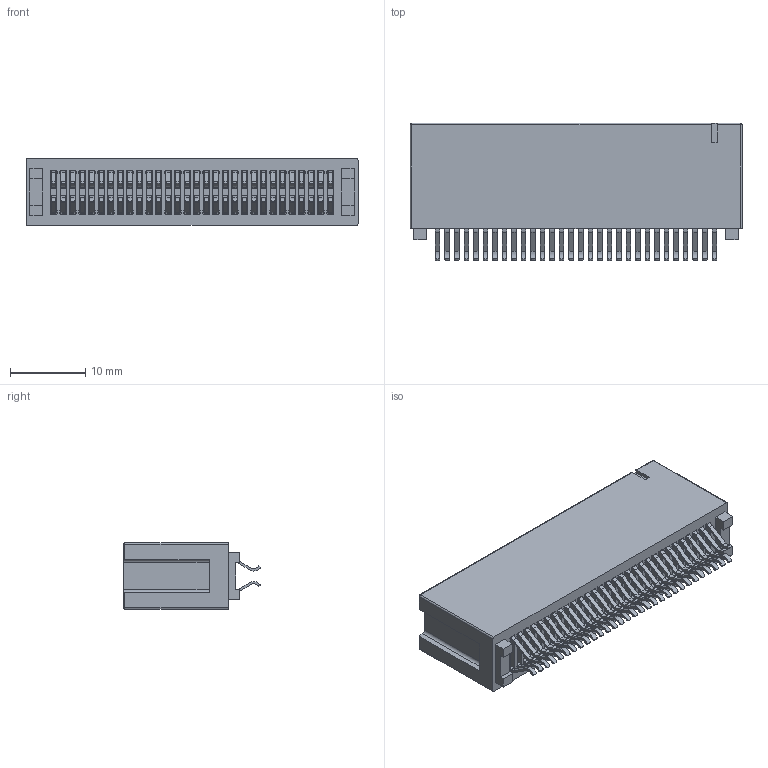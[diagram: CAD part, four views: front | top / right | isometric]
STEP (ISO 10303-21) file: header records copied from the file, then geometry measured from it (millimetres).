
FILE_DESCRIPTION (( 'STEP AP203' ), '1' );
FILE_NAME ('302-060-656-201.STEP', '2024-04-06T05:33:46', ( '' ), ( '' ), 'SwSTEP 2.0', 'SolidWorks 2023', '' );
FILE_SCHEMA (( 'CONFIG_CONTROL_DESIGN' ));
Length unit declared in the file: millimetre
Products named in the file (3): 302-060-656-201; HSG_Vertical HSG; Contact_302-290-X56
Assembly tree (61 placements, depth 2):
  302-060-656-201
    HSG_Vertical HSG
    Contact_302-290-X56  x60
Bounding box: 44.2 x 18.3 x 8.88 mm (x, y, z)
Volume: 3474.7 mm3; surface area: 9399 mm2
Topology: 61 solids, 61 shells, 2916 faces, 8688 edges, 5744 vertices
Faces by surface type: plane 1939, cylinder 973, sphere 4
Entity records: 24195 total; most frequent: ORIENTED_EDGE 4152, CARTESIAN_POINT 4094, DIRECTION 3366, EDGE_CURVE 2076, VECTOR 2018, LINE 2018, VERTEX_POINT 1378, AXIS2_PLACEMENT_3D 674
